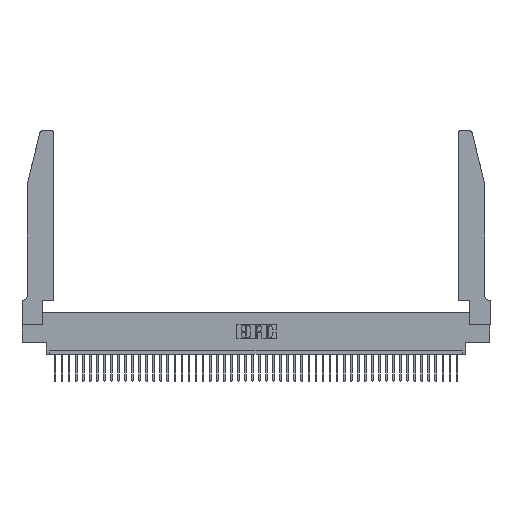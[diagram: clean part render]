
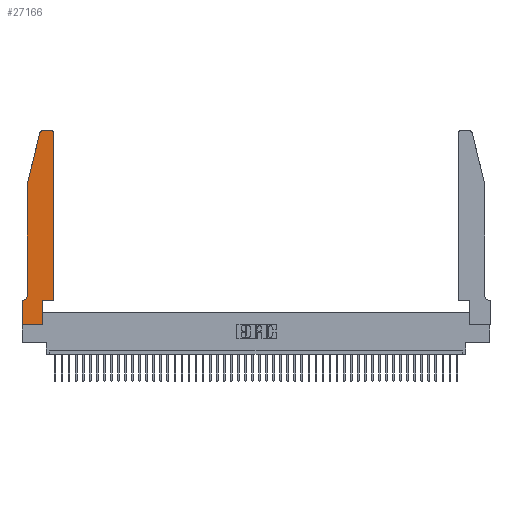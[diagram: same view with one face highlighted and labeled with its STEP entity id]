
A CAD part, top view. The second image highlights one B-rep face of the part: STEP entity #27166.
In plain terms, the highlighted planar face has unit normal (0, 0, 1).
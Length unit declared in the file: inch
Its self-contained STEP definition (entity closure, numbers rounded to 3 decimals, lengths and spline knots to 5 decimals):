
#70 = VERTEX_POINT ( 'NONE', #32858 ) ;
#1416 = VERTEX_POINT ( 'NONE', #34850 ) ;
#2930 = LINE ( 'NONE', #43416, #37647 ) ;
#3319 = CIRCLE ( 'NONE', #5796, 0.03 ) ;
#3592 = EDGE_CURVE ( 'NONE', #15917, #35401, #41215, .T. ) ;
#4184 = VERTEX_POINT ( 'NONE', #37064 ) ;
#4370 = VECTOR ( 'NONE', #35164, 39.37008 ) ;
#4536 = ORIENTED_EDGE ( 'NONE', *, *, #30781, .T. ) ;
#4648 = ORIENTED_EDGE ( 'NONE', *, *, #12177, .T. ) ;
#5144 = VECTOR ( 'NONE', #30158, 39.37008 ) ;
#5486 = EDGE_CURVE ( 'NONE', #17592, #70, #3319, .T. ) ;
#5796 = AXIS2_PLACEMENT_3D ( 'NONE', #10672, #28619, #44425 ) ;
#6006 = CARTESIAN_POINT ( 'NONE',  ( 0.0755, 2., 0.37 ) ) ;
#7610 = DIRECTION ( 'NONE',  ( 0., 0., -1. ) ) ;
#7976 = EDGE_CURVE ( 'NONE', #9580, #4184, #45124, .T. ) ;
#8535 = EDGE_CURVE ( 'NONE', #32069, #32719, #20924, .T. ) ;
#8612 = CARTESIAN_POINT ( 'NONE',  ( 0.2865, 0.35, 0.37 ) ) ;
#8665 = VECTOR ( 'NONE', #22502, 39.37008 ) ;
#9580 = VERTEX_POINT ( 'NONE', #27512 ) ;
#10259 = ORIENTED_EDGE ( 'NONE', *, *, #35985, .T. ) ;
#10587 = CARTESIAN_POINT ( 'NONE',  ( 0.4505, 0.35, 0.37 ) ) ;
#10672 = CARTESIAN_POINT ( 'NONE',  ( 0.284, 2.72, 0.37 ) ) ;
#11860 = CIRCLE ( 'NONE', #46048, 0.07 ) ;
#12177 = EDGE_CURVE ( 'NONE', #41642, #1416, #44607, .T. ) ;
#13186 = LINE ( 'NONE', #24517, #41166 ) ;
#13464 = DIRECTION ( 'NONE',  ( 1., 0., 0. ) ) ;
#13674 = AXIS2_PLACEMENT_3D ( 'NONE', #24445, #38937, #27914 ) ;
#13867 = PLANE ( 'NONE',  #13674 ) ;
#15828 = EDGE_CURVE ( 'NONE', #32719, #41642, #18408, .T. ) ;
#15917 = VERTEX_POINT ( 'NONE', #6006 ) ;
#17338 = DIRECTION ( 'NONE',  ( 0., 0., 1. ) ) ;
#17592 = VERTEX_POINT ( 'NONE', #31266 ) ;
#17748 = CARTESIAN_POINT ( 'NONE',  ( 0.4505, 0.35, 0.37 ) ) ;
#18408 = LINE ( 'NONE', #10587, #36419 ) ;
#18897 = DIRECTION ( 'NONE',  ( -1., 0., 0. ) ) ;
#20239 = EDGE_CURVE ( 'NONE', #4184, #32069, #13186, .T. ) ;
#20274 = EDGE_CURVE ( 'NONE', #1416, #31823, #31077, .T. ) ;
#20924 = LINE ( 'NONE', #46266, #38915 ) ;
#21152 = CARTESIAN_POINT ( 'NONE',  ( 0.4505, 0.35, 0.37 ) ) ;
#21914 = ORIENTED_EDGE ( 'NONE', *, *, #20274, .T. ) ;
#22502 = DIRECTION ( 'NONE',  ( 0., -1., 0. ) ) ;
#24445 = CARTESIAN_POINT ( 'NONE',  ( 0., 0.35, 0.37 ) ) ;
#24517 = CARTESIAN_POINT ( 'NONE',  ( 0., 0., 0.37 ) ) ;
#24638 = CARTESIAN_POINT ( 'NONE',  ( 0.4205, 2.75, 0.37 ) ) ;
#25199 = VERTEX_POINT ( 'NONE', #29205 ) ;
#26137 = CARTESIAN_POINT ( 'NONE',  ( 0.2865, 0., 0.37 ) ) ;
#27166 = ADVANCED_FACE ( 'NONE', ( #29888 ), #13867, .T. ) ;
#27512 = CARTESIAN_POINT ( 'NONE',  ( 0., 0.35, 0.37 ) ) ;
#27914 = DIRECTION ( 'NONE',  ( 1., 0., 0. ) ) ;
#28288 = VECTOR ( 'NONE', #38235, 39.37008 ) ;
#28375 = EDGE_CURVE ( 'NONE', #35401, #25199, #11860, .T. ) ;
#28390 = EDGE_LOOP ( 'NONE', ( #10259, #45507, #4536, #28655, #42093, #33147, #40289, #29789, #39819, #30639, #4648, #21914 ) ) ;
#28619 = DIRECTION ( 'NONE',  ( 0., 0., 1. ) ) ;
#28655 = ORIENTED_EDGE ( 'NONE', *, *, #3592, .T. ) ;
#29013 = CARTESIAN_POINT ( 'NONE',  ( 0.0055, 0.42, 0.37 ) ) ;
#29205 = CARTESIAN_POINT ( 'NONE',  ( 0.0055, 0.35, 0.37 ) ) ;
#29789 = ORIENTED_EDGE ( 'NONE', *, *, #20239, .T. ) ;
#29888 = FACE_OUTER_BOUND ( 'NONE', #28390, .T. ) ;
#30158 = DIRECTION ( 'NONE',  ( -1., 0., 0. ) ) ;
#30639 = ORIENTED_EDGE ( 'NONE', *, *, #15828, .T. ) ;
#30781 = EDGE_CURVE ( 'NONE', #70, #15917, #32397, .T. ) ;
#31077 = CIRCLE ( 'NONE', #42247, 0.03 ) ;
#31266 = CARTESIAN_POINT ( 'NONE',  ( 0.284, 2.75, 0.37 ) ) ;
#31568 = DIRECTION ( 'NONE',  ( 0., 1., 0. ) ) ;
#31823 = VERTEX_POINT ( 'NONE', #24638 ) ;
#32069 = VERTEX_POINT ( 'NONE', #26137 ) ;
#32397 = LINE ( 'NONE', #45648, #4370 ) ;
#32482 = CARTESIAN_POINT ( 'NONE',  ( 0., 0., 0.37 ) ) ;
#32719 = VERTEX_POINT ( 'NONE', #8612 ) ;
#32858 = CARTESIAN_POINT ( 'NONE',  ( 0.25487, 2.72718, 0.37 ) ) ;
#33147 = ORIENTED_EDGE ( 'NONE', *, *, #35231, .T. ) ;
#34850 = CARTESIAN_POINT ( 'NONE',  ( 0.4505, 2.72, 0.37 ) ) ;
#35125 = VECTOR ( 'NONE', #31568, 39.37008 ) ;
#35164 = DIRECTION ( 'NONE',  ( -0.239, -0.971, 0. ) ) ;
#35231 = EDGE_CURVE ( 'NONE', #25199, #9580, #2930, .T. ) ;
#35401 = VERTEX_POINT ( 'NONE', #44500 ) ;
#35985 = EDGE_CURVE ( 'NONE', #31823, #17592, #40422, .T. ) ;
#36419 = VECTOR ( 'NONE', #39371, 39.37008 ) ;
#37064 = CARTESIAN_POINT ( 'NONE',  ( 0., 0., 0.37 ) ) ;
#37647 = VECTOR ( 'NONE', #18897, 39.37008 ) ;
#38235 = DIRECTION ( 'NONE',  ( 0., -1., 0. ) ) ;
#38767 = DIRECTION ( 'NONE',  ( 0., 1., 0. ) ) ;
#38915 = VECTOR ( 'NONE', #38767, 39.37008 ) ;
#38937 = DIRECTION ( 'NONE',  ( 0., 0., 1. ) ) ;
#39371 = DIRECTION ( 'NONE',  ( 1., 0., 0. ) ) ;
#39819 = ORIENTED_EDGE ( 'NONE', *, *, #8535, .T. ) ;
#39856 = DIRECTION ( 'NONE',  ( -1., 0., 0. ) ) ;
#40289 = ORIENTED_EDGE ( 'NONE', *, *, #7976, .T. ) ;
#40422 = LINE ( 'NONE', #41494, #5144 ) ;
#41166 = VECTOR ( 'NONE', #13464, 39.37008 ) ;
#41215 = LINE ( 'NONE', #41350, #28288 ) ;
#41350 = CARTESIAN_POINT ( 'NONE',  ( 0.0755, 2., 0.37 ) ) ;
#41494 = CARTESIAN_POINT ( 'NONE',  ( 0.2605, 2.75, 0.37 ) ) ;
#41642 = VERTEX_POINT ( 'NONE', #21152 ) ;
#42093 = ORIENTED_EDGE ( 'NONE', *, *, #28375, .T. ) ;
#42247 = AXIS2_PLACEMENT_3D ( 'NONE', #46351, #17338, #42313 ) ;
#42313 = DIRECTION ( 'NONE',  ( 1., 0., 0. ) ) ;
#43416 = CARTESIAN_POINT ( 'NONE',  ( 0.0755, 0.35, 0.37 ) ) ;
#44425 = DIRECTION ( 'NONE',  ( 1., 0., 0. ) ) ;
#44500 = CARTESIAN_POINT ( 'NONE',  ( 0.0755, 0.42, 0.37 ) ) ;
#44607 = LINE ( 'NONE', #17748, #35125 ) ;
#45124 = LINE ( 'NONE', #32482, #8665 ) ;
#45507 = ORIENTED_EDGE ( 'NONE', *, *, #5486, .T. ) ;
#45648 = CARTESIAN_POINT ( 'NONE',  ( 0.0755, 2., 0.37 ) ) ;
#46048 = AXIS2_PLACEMENT_3D ( 'NONE', #29013, #7610, #39856 ) ;
#46266 = CARTESIAN_POINT ( 'NONE',  ( 0.2865, 0.35, 0.37 ) ) ;
#46351 = CARTESIAN_POINT ( 'NONE',  ( 0.4205, 2.72, 0.37 ) ) ;
